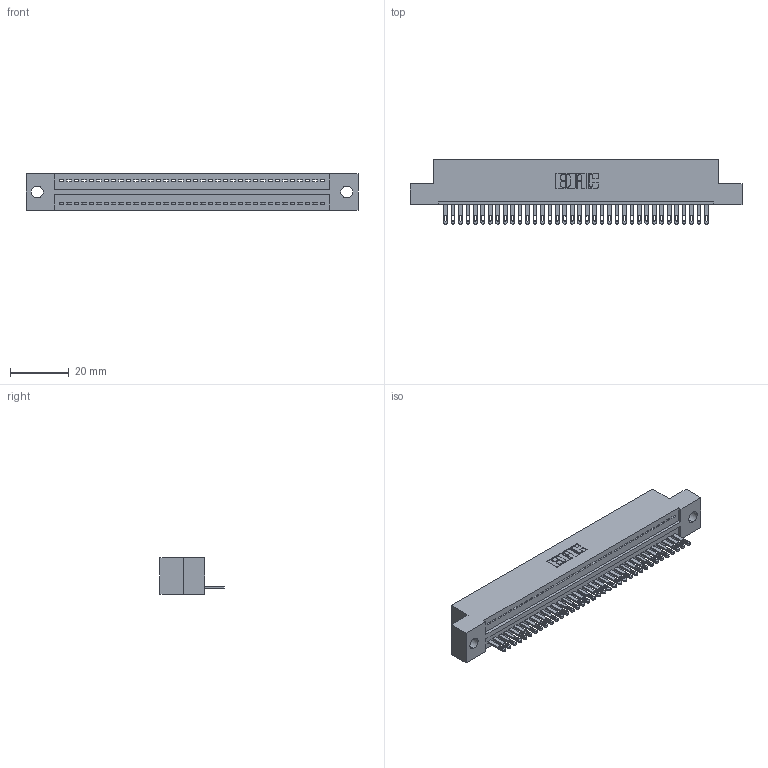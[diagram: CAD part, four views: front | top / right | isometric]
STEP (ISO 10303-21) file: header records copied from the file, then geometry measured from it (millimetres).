
FILE_DESCRIPTION (( 'STEP AP203' ), '1' );
FILE_NAME ('325-036-500-109.STEP', '2020-02-24T20:23:15', ( '' ), ( '' ), 'SwSTEP 2.0', 'SolidWorks 2016', '' );
FILE_SCHEMA (( 'CONFIG_CONTROL_DESIGN' ));
Length unit declared in the file: inch
Products named in the file (3): 325 Part_.160 TH; 325-036-500-109; 325-292-001_325-293-100
Assembly tree (37 placements, depth 2):
  325-036-500-109
    325 Part_.160 TH
    325-292-001_325-293-100  x36
Bounding box: 113.16 x 21.84 x 12.45 mm (x, y, z)
Volume: 14109.7 mm3; surface area: 15293.1 mm2
Topology: 37 solids, 37 shells, 2058 faces, 6359 edges, 4238 vertices
Faces by surface type: plane 1366, cylinder 692
Entity records: 22717 total; most frequent: CARTESIAN_POINT 3926, ORIENTED_EDGE 3898, DIRECTION 3325, EDGE_CURVE 1949, LINE 1817, VECTOR 1817, VERTEX_POINT 1298, AXIS2_PLACEMENT_3D 754
